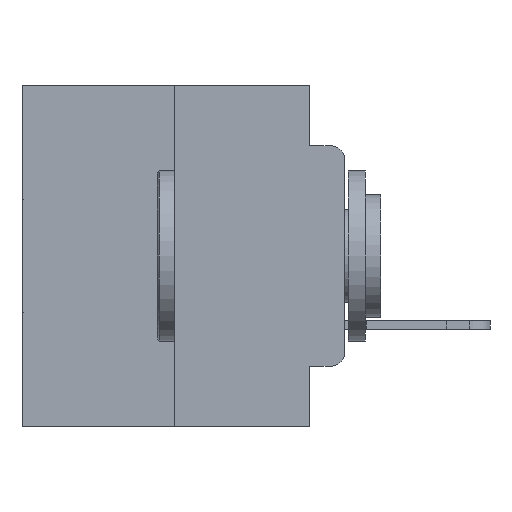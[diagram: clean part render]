
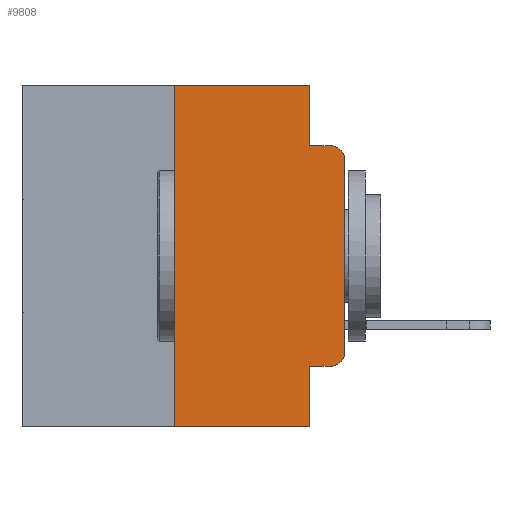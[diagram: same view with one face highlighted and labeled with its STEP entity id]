
A CAD part, left-side view. The second image highlights one B-rep face of the part: STEP entity #9808.
In plain terms, the highlighted planar face has unit normal (-1, 0, 0).
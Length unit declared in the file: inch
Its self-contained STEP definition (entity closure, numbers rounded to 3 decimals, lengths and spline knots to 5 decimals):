
#57 = CARTESIAN_POINT ( 'NONE',  ( 0., 0.473, 0. ) ) ;
#319 = CARTESIAN_POINT ( 'NONE',  ( 0., 0.051, -0.0885 ) ) ;
#867 = CARTESIAN_POINT ( 'NONE',  ( 0., 0.02, -0.1085 ) ) ;
#1323 = CARTESIAN_POINT ( 'NONE',  ( 0., 0.051, 0. ) ) ;
#1422 = VECTOR ( 'NONE', #7353, 39.37008 ) ;
#2055 = VERTEX_POINT ( 'NONE', #319 ) ;
#2257 = CARTESIAN_POINT ( 'NONE',  ( 0., 0., -0.3915 ) ) ;
#2942 = ORIENTED_EDGE ( 'NONE', *, *, #10553, .T. ) ;
#4169 = CARTESIAN_POINT ( 'NONE',  ( 0., 0.02, -0.3915 ) ) ;
#4235 = EDGE_CURVE ( 'NONE', #25849, #16882, #18631, .T. ) ;
#4458 = LINE ( 'NONE', #10360, #15729 ) ;
#4557 = EDGE_CURVE ( 'NONE', #5913, #21443, #15989, .T. ) ;
#4645 = DIRECTION ( 'NONE',  ( 0., -1., 0. ) ) ;
#5226 = VERTEX_POINT ( 'NONE', #2257 ) ;
#5839 = CARTESIAN_POINT ( 'NONE',  ( 0., 0.051, -0.4115 ) ) ;
#5913 = VERTEX_POINT ( 'NONE', #19803 ) ;
#6072 = ORIENTED_EDGE ( 'NONE', *, *, #21292, .F. ) ;
#6134 = CARTESIAN_POINT ( 'NONE',  ( 0., 0.25, 0. ) ) ;
#6513 = CARTESIAN_POINT ( 'NONE',  ( 0., 0.051, 0. ) ) ;
#7230 = LINE ( 'NONE', #18450, #1422 ) ;
#7353 = DIRECTION ( 'NONE',  ( 0., 0., -1. ) ) ;
#7485 = VECTOR ( 'NONE', #4645, 39.37008 ) ;
#7614 = CARTESIAN_POINT ( 'NONE',  ( 0., 0., -0.1085 ) ) ;
#7856 = DIRECTION ( 'NONE',  ( 0., -1., 0. ) ) ;
#7950 = AXIS2_PLACEMENT_3D ( 'NONE', #57, #21603, #21880 ) ;
#8288 = VECTOR ( 'NONE', #7856, 39.37008 ) ;
#8345 = CIRCLE ( 'NONE', #9196, 0.02 ) ;
#8399 = AXIS2_PLACEMENT_3D ( 'NONE', #867, #24952, #22691 ) ;
#8408 = CARTESIAN_POINT ( 'NONE',  ( 0., 0.051, -0.4115 ) ) ;
#8632 = VERTEX_POINT ( 'NONE', #25441 ) ;
#8643 = DIRECTION ( 'NONE',  ( -1., 0., 0. ) ) ;
#8736 = EDGE_CURVE ( 'NONE', #19072, #2055, #17613, .T. ) ;
#9196 = AXIS2_PLACEMENT_3D ( 'NONE', #4169, #8643, #23695 ) ;
#9287 = ORIENTED_EDGE ( 'NONE', *, *, #26099, .T. ) ;
#9808 = ADVANCED_FACE ( 'NONE', ( #23749 ), #28147, .F. ) ;
#10110 = EDGE_CURVE ( 'NONE', #2055, #16882, #17537, .T. ) ;
#10360 = CARTESIAN_POINT ( 'NONE',  ( 0., 0.473, 0. ) ) ;
#10553 = EDGE_CURVE ( 'NONE', #10686, #8632, #27063, .T. ) ;
#10686 = VERTEX_POINT ( 'NONE', #8408 ) ;
#10809 = CARTESIAN_POINT ( 'NONE',  ( 0., 0., 0. ) ) ;
#11046 = ORIENTED_EDGE ( 'NONE', *, *, #4557, .F. ) ;
#11185 = CARTESIAN_POINT ( 'NONE',  ( 0., 0.051, -0.0885 ) ) ;
#11421 = EDGE_CURVE ( 'NONE', #21443, #19072, #4458, .T. ) ;
#11505 = CARTESIAN_POINT ( 'NONE',  ( 0., 0.051, -0.5 ) ) ;
#12726 = ORIENTED_EDGE ( 'NONE', *, *, #11421, .F. ) ;
#13173 = EDGE_CURVE ( 'NONE', #5913, #25591, #28323, .T. ) ;
#13423 = CARTESIAN_POINT ( 'NONE',  ( 0., 0.473, -0.5 ) ) ;
#14657 = DIRECTION ( 'NONE',  ( 0., -1., 0. ) ) ;
#15217 = DIRECTION ( 'NONE',  ( 0., 0., 1. ) ) ;
#15504 = DIRECTION ( 'NONE',  ( 0., -1., 0. ) ) ;
#15729 = VECTOR ( 'NONE', #14657, 39.37008 ) ;
#15989 = LINE ( 'NONE', #6134, #21496 ) ;
#16622 = CARTESIAN_POINT ( 'NONE',  ( 0., 0.25, 0. ) ) ;
#16882 = VERTEX_POINT ( 'NONE', #25570 ) ;
#16883 = VECTOR ( 'NONE', #15504, 39.37008 ) ;
#17537 = LINE ( 'NONE', #11185, #16883 ) ;
#17613 = LINE ( 'NONE', #6513, #23799 ) ;
#18450 = CARTESIAN_POINT ( 'NONE',  ( 0., 0.051, 0. ) ) ;
#18470 = ORIENTED_EDGE ( 'NONE', *, *, #22758, .T. ) ;
#18631 = CIRCLE ( 'NONE', #8399, 0.02 ) ;
#19022 = ORIENTED_EDGE ( 'NONE', *, *, #10110, .F. ) ;
#19072 = VERTEX_POINT ( 'NONE', #1323 ) ;
#19468 = VECTOR ( 'NONE', #15217, 39.37008 ) ;
#19803 = CARTESIAN_POINT ( 'NONE',  ( 0., 0.25, -0.5 ) ) ;
#21292 = EDGE_CURVE ( 'NONE', #10686, #25591, #7230, .T. ) ;
#21443 = VERTEX_POINT ( 'NONE', #16622 ) ;
#21496 = VECTOR ( 'NONE', #26003, 39.37008 ) ;
#21539 = LINE ( 'NONE', #10809, #19468 ) ;
#21603 = DIRECTION ( 'NONE',  ( 1., 0., 0. ) ) ;
#21880 = DIRECTION ( 'NONE',  ( 0., 0., -1. ) ) ;
#22691 = DIRECTION ( 'NONE',  ( 0., 0., -1. ) ) ;
#22758 = EDGE_CURVE ( 'NONE', #5226, #25849, #21539, .T. ) ;
#23695 = DIRECTION ( 'NONE',  ( 0., 0., -1. ) ) ;
#23749 = FACE_OUTER_BOUND ( 'NONE', #25790, .T. ) ;
#23799 = VECTOR ( 'NONE', #25916, 39.37008 ) ;
#24952 = DIRECTION ( 'NONE',  ( -1., 0., 0. ) ) ;
#24999 = ORIENTED_EDGE ( 'NONE', *, *, #13173, .T. ) ;
#25186 = ORIENTED_EDGE ( 'NONE', *, *, #4235, .T. ) ;
#25441 = CARTESIAN_POINT ( 'NONE',  ( 0., 0.02, -0.4115 ) ) ;
#25570 = CARTESIAN_POINT ( 'NONE',  ( 0., 0.02, -0.0885 ) ) ;
#25591 = VERTEX_POINT ( 'NONE', #11505 ) ;
#25790 = EDGE_LOOP ( 'NONE', ( #18470, #25186, #19022, #26488, #12726, #11046, #24999, #6072, #2942, #9287 ) ) ;
#25849 = VERTEX_POINT ( 'NONE', #7614 ) ;
#25916 = DIRECTION ( 'NONE',  ( 0., 0., -1. ) ) ;
#26003 = DIRECTION ( 'NONE',  ( 0., 0., 1. ) ) ;
#26099 = EDGE_CURVE ( 'NONE', #8632, #5226, #8345, .T. ) ;
#26488 = ORIENTED_EDGE ( 'NONE', *, *, #8736, .F. ) ;
#27063 = LINE ( 'NONE', #5839, #8288 ) ;
#28147 = PLANE ( 'NONE',  #7950 ) ;
#28323 = LINE ( 'NONE', #13423, #7485 ) ;
